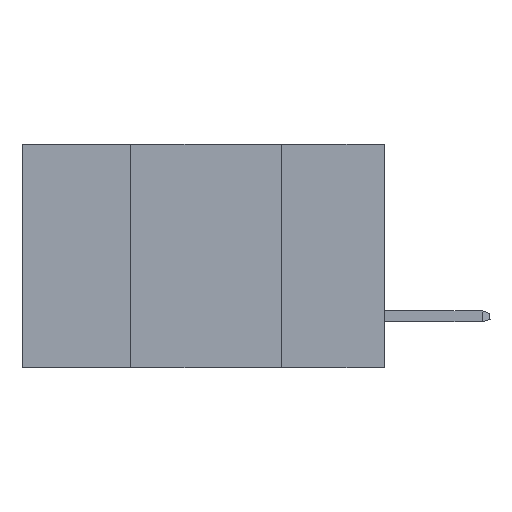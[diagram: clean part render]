
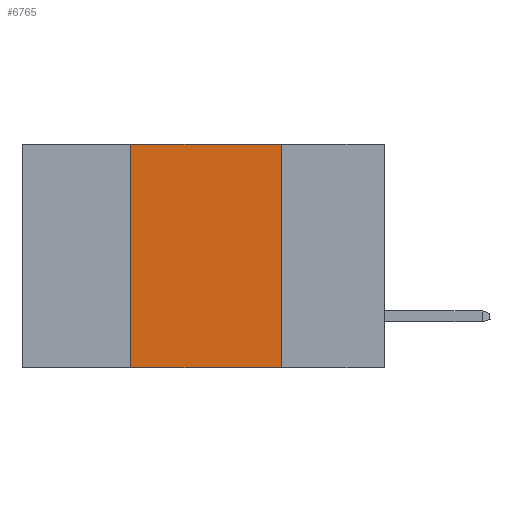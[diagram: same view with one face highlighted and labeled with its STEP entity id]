
A CAD part, left-side view. The second image highlights one B-rep face of the part: STEP entity #6765.
In plain terms, the highlighted planar face has unit normal (-1, 0, 0).
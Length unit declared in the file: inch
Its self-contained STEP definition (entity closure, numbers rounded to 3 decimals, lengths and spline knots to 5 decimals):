
#2866 = LINE ( 'NONE', #3163, #28892 ) ;
#3163 = CARTESIAN_POINT ( 'NONE',  ( 0., 0.6, 0. ) ) ;
#5174 = DIRECTION ( 'NONE',  ( 0., 0., -1. ) ) ;
#5255 = CARTESIAN_POINT ( 'NONE',  ( 0., 0.17, -0.37 ) ) ;
#6397 = VECTOR ( 'NONE', #5174, 39.37008 ) ;
#6765 = ADVANCED_FACE ( 'NONE', ( #25823 ), #19642, .F. ) ;
#8993 = AXIS2_PLACEMENT_3D ( 'NONE', #22019, #10196, #24518 ) ;
#10196 = DIRECTION ( 'NONE',  ( 1., 0., 0. ) ) ;
#10884 = CARTESIAN_POINT ( 'NONE',  ( 0., 0.42, -0.37 ) ) ;
#10899 = ORIENTED_EDGE ( 'NONE', *, *, #12785, .F. ) ;
#11204 = LINE ( 'NONE', #12303, #6397 ) ;
#12303 = CARTESIAN_POINT ( 'NONE',  ( 0., 0.17, 0. ) ) ;
#12785 = EDGE_CURVE ( 'NONE', #29684, #19955, #11204, .T. ) ;
#12996 = DIRECTION ( 'NONE',  ( 0., -1., 0. ) ) ;
#14053 = DIRECTION ( 'NONE',  ( 0., -1., 0. ) ) ;
#14664 = EDGE_LOOP ( 'NONE', ( #10899, #24249, #20105, #17635 ) ) ;
#15021 = CARTESIAN_POINT ( 'NONE',  ( 0., 0.17, 0. ) ) ;
#15264 = DIRECTION ( 'NONE',  ( 0., 0., 1. ) ) ;
#16229 = LINE ( 'NONE', #29654, #27382 ) ;
#17635 = ORIENTED_EDGE ( 'NONE', *, *, #29224, .T. ) ;
#19343 = VECTOR ( 'NONE', #14053, 39.37008 ) ;
#19642 = PLANE ( 'NONE',  #8993 ) ;
#19955 = VERTEX_POINT ( 'NONE', #5255 ) ;
#20105 = ORIENTED_EDGE ( 'NONE', *, *, #22643, .F. ) ;
#22019 = CARTESIAN_POINT ( 'NONE',  ( 0., 0.6, 0. ) ) ;
#22610 = EDGE_CURVE ( 'NONE', #27325, #29684, #2866, .T. ) ;
#22643 = EDGE_CURVE ( 'NONE', #27770, #27325, #16229, .T. ) ;
#23299 = CARTESIAN_POINT ( 'NONE',  ( 0., 0.6, -0.37 ) ) ;
#24249 = ORIENTED_EDGE ( 'NONE', *, *, #22610, .F. ) ;
#24518 = DIRECTION ( 'NONE',  ( 0., 0., -1. ) ) ;
#25823 = FACE_OUTER_BOUND ( 'NONE', #14664, .T. ) ;
#26194 = CARTESIAN_POINT ( 'NONE',  ( 0., 0.42, 0. ) ) ;
#27169 = LINE ( 'NONE', #23299, #19343 ) ;
#27325 = VERTEX_POINT ( 'NONE', #26194 ) ;
#27382 = VECTOR ( 'NONE', #15264, 39.37008 ) ;
#27770 = VERTEX_POINT ( 'NONE', #10884 ) ;
#28892 = VECTOR ( 'NONE', #12996, 39.37008 ) ;
#29224 = EDGE_CURVE ( 'NONE', #27770, #19955, #27169, .T. ) ;
#29654 = CARTESIAN_POINT ( 'NONE',  ( 0., 0.42, 0. ) ) ;
#29684 = VERTEX_POINT ( 'NONE', #15021 ) ;
